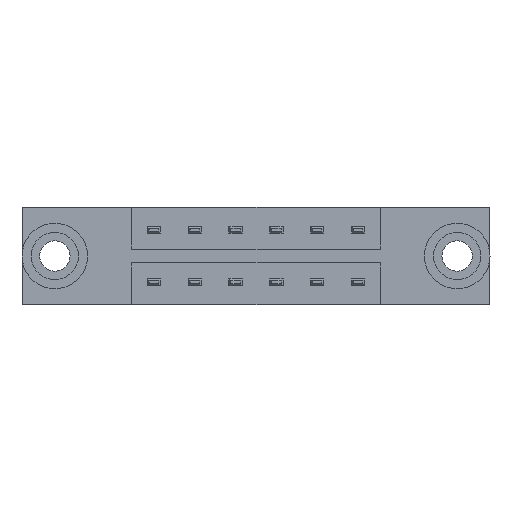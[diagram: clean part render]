
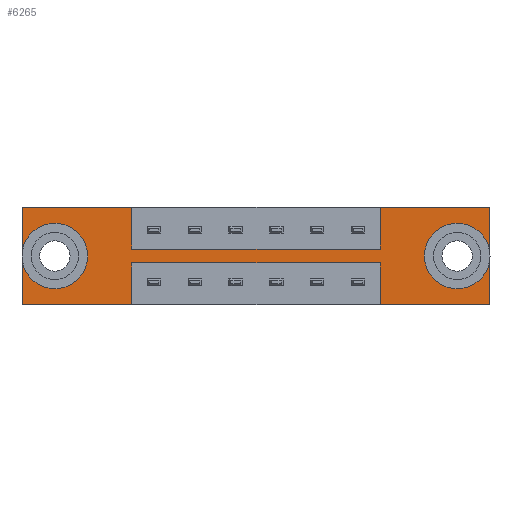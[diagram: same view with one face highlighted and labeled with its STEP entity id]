
A CAD part, front view. The second image highlights one B-rep face of the part: STEP entity #6265.
In plain terms, the highlighted planar face has unit normal (0, -1, 0).
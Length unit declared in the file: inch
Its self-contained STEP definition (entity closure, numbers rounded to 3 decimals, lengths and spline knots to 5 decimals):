
#4 = VERTEX_POINT ( 'NONE', #676 ) ;
#12 = VERTEX_POINT ( 'NONE', #8236 ) ;
#66 = CARTESIAN_POINT ( 'NONE',  ( 1.659, 0., -0.107 ) ) ;
#138 = VERTEX_POINT ( 'NONE', #8378 ) ;
#162 = FACE_OUTER_BOUND ( 'NONE', #2110, .T. ) ;
#239 = VERTEX_POINT ( 'NONE', #6036 ) ;
#261 = LINE ( 'NONE', #3052, #8658 ) ;
#282 = VECTOR ( 'NONE', #8904, 39.37008 ) ;
#360 = CIRCLE ( 'NONE', #6899, 0.078 ) ;
#406 = DIRECTION ( 'NONE',  ( 0., 1., 0. ) ) ;
#445 = CARTESIAN_POINT ( 'NONE',  ( 1.659, 0., -0.185 ) ) ;
#676 = CARTESIAN_POINT ( 'NONE',  ( 0., 0., 0. ) ) ;
#736 = LINE ( 'NONE', #6848, #8640 ) ;
#966 = ORIENTED_EDGE ( 'NONE', *, *, #5956, .F. ) ;
#978 = EDGE_CURVE ( 'NONE', #5693, #7225, #6147, .T. ) ;
#1009 = VERTEX_POINT ( 'NONE', #7072 ) ;
#1139 = LINE ( 'NONE', #3923, #2235 ) ;
#1207 = LINE ( 'NONE', #3212, #5488 ) ;
#1279 = DIRECTION ( 'NONE',  ( 0., 0., -1. ) ) ;
#1307 = VERTEX_POINT ( 'NONE', #7599 ) ;
#1310 = LINE ( 'NONE', #4039, #4093 ) ;
#1364 = CARTESIAN_POINT ( 'NONE',  ( 0.4175, 0., -0.1585 ) ) ;
#1386 = AXIS2_PLACEMENT_3D ( 'NONE', #1815, #4590, #6771 ) ;
#1422 = LINE ( 'NONE', #6332, #3997 ) ;
#1585 = FACE_BOUND ( 'NONE', #3664, .T. ) ;
#1705 = DIRECTION ( 'NONE',  ( 0., 1., 0. ) ) ;
#1747 = ORIENTED_EDGE ( 'NONE', *, *, #8753, .F. ) ;
#1815 = CARTESIAN_POINT ( 'NONE',  ( 1.659, 0., -0.185 ) ) ;
#2005 = CARTESIAN_POINT ( 'NONE',  ( 0.125, 0., -0.107 ) ) ;
#2040 = AXIS2_PLACEMENT_3D ( 'NONE', #3007, #2274, #6314 ) ;
#2085 = VERTEX_POINT ( 'NONE', #7407 ) ;
#2110 = EDGE_LOOP ( 'NONE', ( #1747, #7454, #6603, #2914, #7302, #4986, #4555, #966, #2206, #5112, #8306, #6427 ) ) ;
#2176 = FACE_BOUND ( 'NONE', #4546, .T. ) ;
#2202 = EDGE_CURVE ( 'NONE', #138, #1009, #1422, .T. ) ;
#2206 = ORIENTED_EDGE ( 'NONE', *, *, #6051, .F. ) ;
#2235 = VECTOR ( 'NONE', #5271, 39.37008 ) ;
#2274 = DIRECTION ( 'NONE',  ( 0., -1., 0. ) ) ;
#2306 = CARTESIAN_POINT ( 'NONE',  ( 0., 0., -0.37 ) ) ;
#2363 = LINE ( 'NONE', #7249, #7143 ) ;
#2465 = ORIENTED_EDGE ( 'NONE', *, *, #5665, .T. ) ;
#2498 = DIRECTION ( 'NONE',  ( 0., 0., 1. ) ) ;
#2598 = CARTESIAN_POINT ( 'NONE',  ( 1.784, 0., 0. ) ) ;
#2679 = DIRECTION ( 'NONE',  ( -1., 0., 0. ) ) ;
#2779 = CARTESIAN_POINT ( 'NONE',  ( 0., 0., 0. ) ) ;
#2881 = EDGE_CURVE ( 'NONE', #4613, #5693, #261, .T. ) ;
#2909 = EDGE_CURVE ( 'NONE', #7025, #8395, #3877, .T. ) ;
#2914 = ORIENTED_EDGE ( 'NONE', *, *, #6177, .F. ) ;
#2917 = LINE ( 'NONE', #3705, #7170 ) ;
#3007 = CARTESIAN_POINT ( 'NONE',  ( 0., 0., -0.37 ) ) ;
#3052 = CARTESIAN_POINT ( 'NONE',  ( 0.4175, 0., -0.2115 ) ) ;
#3169 = CARTESIAN_POINT ( 'NONE',  ( 0.125, 0., -0.185 ) ) ;
#3198 = VERTEX_POINT ( 'NONE', #3746 ) ;
#3212 = CARTESIAN_POINT ( 'NONE',  ( 0.4175, 0., -0.2115 ) ) ;
#3262 = DIRECTION ( 'NONE',  ( -1., 0., 0. ) ) ;
#3456 = EDGE_CURVE ( 'NONE', #8395, #7025, #5583, .T. ) ;
#3484 = CARTESIAN_POINT ( 'NONE',  ( 1.784, 0., -0.37 ) ) ;
#3552 = AXIS2_PLACEMENT_3D ( 'NONE', #445, #406, #7511 ) ;
#3650 = VERTEX_POINT ( 'NONE', #3484 ) ;
#3664 = EDGE_LOOP ( 'NONE', ( #4577, #2465 ) ) ;
#3705 = CARTESIAN_POINT ( 'NONE',  ( 0., 0., 0. ) ) ;
#3746 = CARTESIAN_POINT ( 'NONE',  ( 0.125, 0., -0.263 ) ) ;
#3854 = EDGE_CURVE ( 'NONE', #1307, #4613, #1207, .T. ) ;
#3877 = CIRCLE ( 'NONE', #3552, 0.078 ) ;
#3923 = CARTESIAN_POINT ( 'NONE',  ( 0., 0., 0. ) ) ;
#3969 = DIRECTION ( 'NONE',  ( 0., 0., -1. ) ) ;
#3997 = VECTOR ( 'NONE', #4193, 39.37008 ) ;
#4039 = CARTESIAN_POINT ( 'NONE',  ( 0., 0., -0.37 ) ) ;
#4048 = LINE ( 'NONE', #2779, #282 ) ;
#4093 = VECTOR ( 'NONE', #2679, 39.37008 ) ;
#4193 = DIRECTION ( 'NONE',  ( 1., 0., 0. ) ) ;
#4275 = PLANE ( 'NONE',  #2040 ) ;
#4447 = CARTESIAN_POINT ( 'NONE',  ( 1.784, 0., 0. ) ) ;
#4477 = CARTESIAN_POINT ( 'NONE',  ( 0.4175, 0., -0.37 ) ) ;
#4520 = DIRECTION ( 'NONE',  ( 0., 0., 1. ) ) ;
#4546 = EDGE_LOOP ( 'NONE', ( #7735, #8531 ) ) ;
#4555 = ORIENTED_EDGE ( 'NONE', *, *, #6151, .F. ) ;
#4577 = ORIENTED_EDGE ( 'NONE', *, *, #6554, .T. ) ;
#4590 = DIRECTION ( 'NONE',  ( 0., 1., 0. ) ) ;
#4613 = VERTEX_POINT ( 'NONE', #5369 ) ;
#4646 = LINE ( 'NONE', #2598, #7602 ) ;
#4787 = VECTOR ( 'NONE', #1279, 39.37008 ) ;
#4986 = ORIENTED_EDGE ( 'NONE', *, *, #2202, .F. ) ;
#5111 = VERTEX_POINT ( 'NONE', #4447 ) ;
#5112 = ORIENTED_EDGE ( 'NONE', *, *, #978, .F. ) ;
#5271 = DIRECTION ( 'NONE',  ( 0., 0., 1. ) ) ;
#5312 = CARTESIAN_POINT ( 'NONE',  ( 0.125, 0., -0.185 ) ) ;
#5369 = CARTESIAN_POINT ( 'NONE',  ( 0.4175, 0., -0.2115 ) ) ;
#5488 = VECTOR ( 'NONE', #3262, 39.37008 ) ;
#5583 = CIRCLE ( 'NONE', #1386, 0.078 ) ;
#5665 = EDGE_CURVE ( 'NONE', #3198, #5768, #360, .T. ) ;
#5693 = VERTEX_POINT ( 'NONE', #4477 ) ;
#5768 = VERTEX_POINT ( 'NONE', #2005 ) ;
#5820 = DIRECTION ( 'NONE',  ( 0., 0., -1. ) ) ;
#5956 = EDGE_CURVE ( 'NONE', #4, #2085, #2917, .T. ) ;
#6036 = CARTESIAN_POINT ( 'NONE',  ( 1.3665, 0., 0. ) ) ;
#6051 = EDGE_CURVE ( 'NONE', #7225, #4, #1139, .T. ) ;
#6122 = AXIS2_PLACEMENT_3D ( 'NONE', #5312, #6812, #8096 ) ;
#6147 = LINE ( 'NONE', #8919, #8742 ) ;
#6151 = EDGE_CURVE ( 'NONE', #2085, #138, #8952, .T. ) ;
#6177 = EDGE_CURVE ( 'NONE', #239, #5111, #4048, .T. ) ;
#6205 = DIRECTION ( 'NONE',  ( 0., 0., 1. ) ) ;
#6265 = ADVANCED_FACE ( 'NONE', ( #2176, #1585, #162 ), #4275, .T. ) ;
#6314 = DIRECTION ( 'NONE',  ( 0., 0., -1. ) ) ;
#6332 = CARTESIAN_POINT ( 'NONE',  ( 0.4175, 0., -0.1585 ) ) ;
#6426 = EDGE_CURVE ( 'NONE', #1009, #239, #2363, .T. ) ;
#6427 = ORIENTED_EDGE ( 'NONE', *, *, #3854, .F. ) ;
#6554 = EDGE_CURVE ( 'NONE', #5768, #3198, #8883, .T. ) ;
#6603 = ORIENTED_EDGE ( 'NONE', *, *, #7819, .F. ) ;
#6608 = EDGE_CURVE ( 'NONE', #3650, #12, #1310, .T. ) ;
#6771 = DIRECTION ( 'NONE',  ( 0., 0., -1. ) ) ;
#6812 = DIRECTION ( 'NONE',  ( 0., 1., 0. ) ) ;
#6848 = CARTESIAN_POINT ( 'NONE',  ( 1.3665, 0., -0.2115 ) ) ;
#6899 = AXIS2_PLACEMENT_3D ( 'NONE', #3169, #1705, #4520 ) ;
#7025 = VERTEX_POINT ( 'NONE', #8397 ) ;
#7072 = CARTESIAN_POINT ( 'NONE',  ( 1.3665, 0., -0.1585 ) ) ;
#7143 = VECTOR ( 'NONE', #2498, 39.37008 ) ;
#7170 = VECTOR ( 'NONE', #7789, 39.37008 ) ;
#7225 = VERTEX_POINT ( 'NONE', #2306 ) ;
#7249 = CARTESIAN_POINT ( 'NONE',  ( 1.3665, 0., -0.1585 ) ) ;
#7302 = ORIENTED_EDGE ( 'NONE', *, *, #6426, .F. ) ;
#7407 = CARTESIAN_POINT ( 'NONE',  ( 0.4175, 0., 0. ) ) ;
#7454 = ORIENTED_EDGE ( 'NONE', *, *, #6608, .F. ) ;
#7511 = DIRECTION ( 'NONE',  ( 0., 0., -1. ) ) ;
#7599 = CARTESIAN_POINT ( 'NONE',  ( 1.3665, 0., -0.2115 ) ) ;
#7602 = VECTOR ( 'NONE', #3969, 39.37008 ) ;
#7735 = ORIENTED_EDGE ( 'NONE', *, *, #3456, .T. ) ;
#7789 = DIRECTION ( 'NONE',  ( 1., 0., 0. ) ) ;
#7819 = EDGE_CURVE ( 'NONE', #5111, #3650, #4646, .T. ) ;
#8096 = DIRECTION ( 'NONE',  ( 0., 0., 1. ) ) ;
#8236 = CARTESIAN_POINT ( 'NONE',  ( 1.3665, 0., -0.37 ) ) ;
#8248 = DIRECTION ( 'NONE',  ( -1., 0., 0. ) ) ;
#8306 = ORIENTED_EDGE ( 'NONE', *, *, #2881, .F. ) ;
#8378 = CARTESIAN_POINT ( 'NONE',  ( 0.4175, 0., -0.1585 ) ) ;
#8395 = VERTEX_POINT ( 'NONE', #66 ) ;
#8397 = CARTESIAN_POINT ( 'NONE',  ( 1.659, 0., -0.263 ) ) ;
#8531 = ORIENTED_EDGE ( 'NONE', *, *, #2909, .T. ) ;
#8640 = VECTOR ( 'NONE', #6205, 39.37008 ) ;
#8658 = VECTOR ( 'NONE', #5820, 39.37008 ) ;
#8742 = VECTOR ( 'NONE', #8248, 39.37008 ) ;
#8753 = EDGE_CURVE ( 'NONE', #12, #1307, #736, .T. ) ;
#8883 = CIRCLE ( 'NONE', #6122, 0.078 ) ;
#8904 = DIRECTION ( 'NONE',  ( 1., 0., 0. ) ) ;
#8919 = CARTESIAN_POINT ( 'NONE',  ( 0., 0., -0.37 ) ) ;
#8952 = LINE ( 'NONE', #1364, #4787 ) ;
